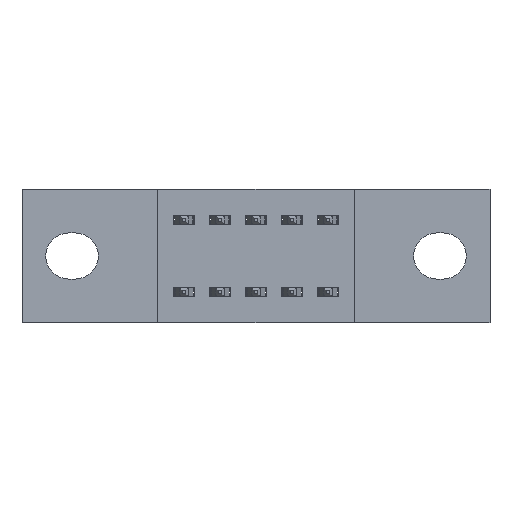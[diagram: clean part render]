
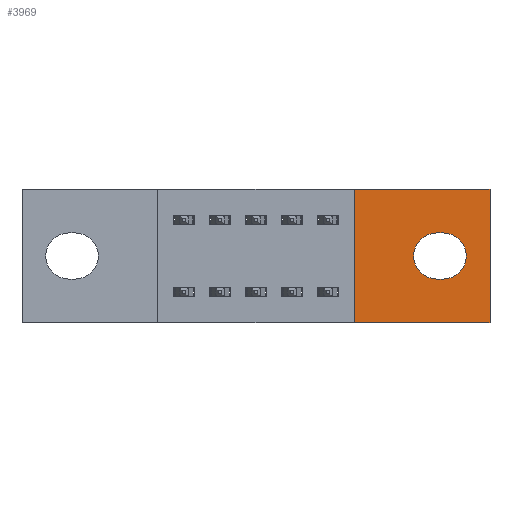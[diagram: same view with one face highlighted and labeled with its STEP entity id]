
A CAD part, front view. The second image highlights one B-rep face of the part: STEP entity #3969.
In plain terms, the highlighted planar face has unit normal (0, -1, 0).
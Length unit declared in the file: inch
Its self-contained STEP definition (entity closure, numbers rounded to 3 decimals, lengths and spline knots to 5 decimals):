
#423 = DIRECTION ( 'NONE',  ( 0., 0., -1. ) ) ;
#455 = PLANE ( 'NONE',  #546 ) ;
#546 = AXIS2_PLACEMENT_3D ( 'NONE', #2658, #928, #423 ) ;
#848 = CARTESIAN_POINT ( 'NONE',  ( 1.3, 0., -0.37 ) ) ;
#928 = DIRECTION ( 'NONE',  ( 0., -1., 0. ) ) ;
#992 = DIRECTION ( 'NONE',  ( 0., 0., -1. ) ) ;
#1018 = DIRECTION ( 'NONE',  ( 0., 1., 0. ) ) ;
#1177 = FACE_BOUND ( 'NONE', #7489, .T. ) ;
#1192 = CARTESIAN_POINT ( 'NONE',  ( 1.17, 0., -0.121 ) ) ;
#1384 = FACE_OUTER_BOUND ( 'NONE', #2013, .T. ) ;
#1455 = VERTEX_POINT ( 'NONE', #4853 ) ;
#1534 = AXIS2_PLACEMENT_3D ( 'NONE', #5815, #2267, #6520 ) ;
#1757 = LINE ( 'NONE', #1192, #3696 ) ;
#2013 = EDGE_LOOP ( 'NONE', ( #4217, #4164, #4060, #3974 ) ) ;
#2069 = CARTESIAN_POINT ( 'NONE',  ( 0., 0., -0.37 ) ) ;
#2267 = DIRECTION ( 'NONE',  ( 0., 1., 0. ) ) ;
#2285 = CARTESIAN_POINT ( 'NONE',  ( 1.152, 0., -0.249 ) ) ;
#2419 = VERTEX_POINT ( 'NONE', #7565 ) ;
#2658 = CARTESIAN_POINT ( 'NONE',  ( 0., 0., -0.37 ) ) ;
#2844 = VERTEX_POINT ( 'NONE', #2285 ) ;
#2952 = VERTEX_POINT ( 'NONE', #7334 ) ;
#2990 = VERTEX_POINT ( 'NONE', #848 ) ;
#3001 = VERTEX_POINT ( 'NONE', #6427 ) ;
#3223 = EDGE_CURVE ( 'NONE', #7941, #2419, #7744, .T. ) ;
#3251 = EDGE_CURVE ( 'NONE', #2419, #2844, #6193, .T. ) ;
#3371 = EDGE_CURVE ( 'NONE', #2844, #7186, #5702, .T. ) ;
#3418 = EDGE_CURVE ( 'NONE', #7186, #7941, #1757, .T. ) ;
#3449 = EDGE_CURVE ( 'NONE', #3001, #1455, #6759, .T. ) ;
#3466 = EDGE_CURVE ( 'NONE', #2990, #3001, #5002, .T. ) ;
#3537 = EDGE_CURVE ( 'NONE', #2952, #2990, #7332, .T. ) ;
#3634 = DIRECTION ( 'NONE',  ( 1., 0., 0. ) ) ;
#3696 = VECTOR ( 'NONE', #3634, 39.37008 ) ;
#3906 = DIRECTION ( 'NONE',  ( 0., 0., -1. ) ) ;
#3915 = CARTESIAN_POINT ( 'NONE',  ( 1.3, 0., 0. ) ) ;
#3969 = ADVANCED_FACE ( 'NONE', ( #1177, #1384 ), #455, .T. ) ;
#3974 = ORIENTED_EDGE ( 'NONE', *, *, #4904, .F. ) ;
#4060 = ORIENTED_EDGE ( 'NONE', *, *, #3537, .F. ) ;
#4164 = ORIENTED_EDGE ( 'NONE', *, *, #3466, .F. ) ;
#4217 = ORIENTED_EDGE ( 'NONE', *, *, #3449, .F. ) ;
#4367 = ORIENTED_EDGE ( 'NONE', *, *, #3418, .T. ) ;
#4381 = ORIENTED_EDGE ( 'NONE', *, *, #3371, .T. ) ;
#4398 = ORIENTED_EDGE ( 'NONE', *, *, #3251, .T. ) ;
#4558 = CARTESIAN_POINT ( 'NONE',  ( 1.17, 0., -0.121 ) ) ;
#4742 = VECTOR ( 'NONE', #6486, 39.37008 ) ;
#4853 = CARTESIAN_POINT ( 'NONE',  ( 0.923, 0., 0. ) ) ;
#4904 = EDGE_CURVE ( 'NONE', #1455, #2952, #6581, .T. ) ;
#5002 = LINE ( 'NONE', #2069, #6419 ) ;
#5702 = CIRCLE ( 'NONE', #5936, 0.064 ) ;
#5766 = CARTESIAN_POINT ( 'NONE',  ( 1.17, 0., -0.249 ) ) ;
#5815 = CARTESIAN_POINT ( 'NONE',  ( 1.17, 0., -0.185 ) ) ;
#5895 = DIRECTION ( 'NONE',  ( 1., 0., 0. ) ) ;
#5936 = AXIS2_PLACEMENT_3D ( 'NONE', #6113, #1018, #992 ) ;
#6113 = CARTESIAN_POINT ( 'NONE',  ( 1.152, 0., -0.185 ) ) ;
#6130 = CARTESIAN_POINT ( 'NONE',  ( 1.152, 0., -0.121 ) ) ;
#6193 = LINE ( 'NONE', #5766, #4742 ) ;
#6194 = ORIENTED_EDGE ( 'NONE', *, *, #3223, .T. ) ;
#6197 = DIRECTION ( 'NONE',  ( -1., 0., 0. ) ) ;
#6398 = VECTOR ( 'NONE', #5895, 39.37008 ) ;
#6419 = VECTOR ( 'NONE', #6197, 39.37008 ) ;
#6427 = CARTESIAN_POINT ( 'NONE',  ( 0.923, 0., -0.37 ) ) ;
#6486 = DIRECTION ( 'NONE',  ( -1., 0., 0. ) ) ;
#6520 = DIRECTION ( 'NONE',  ( 0., 0., -1. ) ) ;
#6581 = LINE ( 'NONE', #6772, #6398 ) ;
#6596 = VECTOR ( 'NONE', #6701, 39.37008 ) ;
#6701 = DIRECTION ( 'NONE',  ( 0., 0., 1. ) ) ;
#6759 = LINE ( 'NONE', #7030, #6596 ) ;
#6772 = CARTESIAN_POINT ( 'NONE',  ( 0., 0., 0. ) ) ;
#7030 = CARTESIAN_POINT ( 'NONE',  ( 0.923, 0., -0.37 ) ) ;
#7183 = VECTOR ( 'NONE', #3906, 39.37008 ) ;
#7186 = VERTEX_POINT ( 'NONE', #6130 ) ;
#7332 = LINE ( 'NONE', #3915, #7183 ) ;
#7334 = CARTESIAN_POINT ( 'NONE',  ( 1.3, 0., 0. ) ) ;
#7489 = EDGE_LOOP ( 'NONE', ( #6194, #4398, #4381, #4367 ) ) ;
#7565 = CARTESIAN_POINT ( 'NONE',  ( 1.17, 0., -0.249 ) ) ;
#7744 = CIRCLE ( 'NONE', #1534, 0.064 ) ;
#7941 = VERTEX_POINT ( 'NONE', #4558 ) ;
